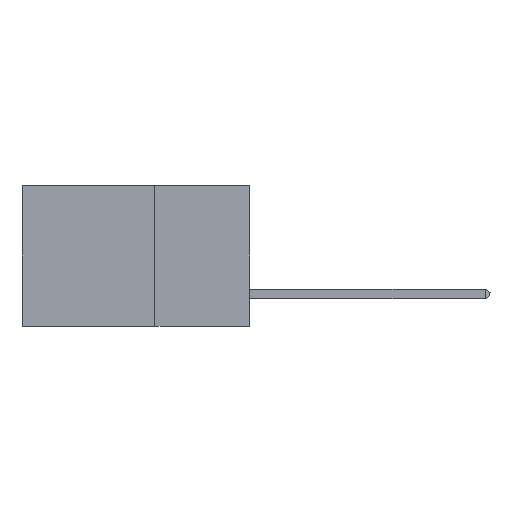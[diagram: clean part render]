
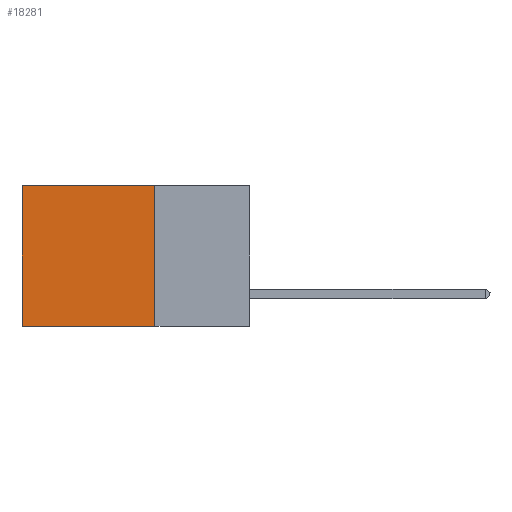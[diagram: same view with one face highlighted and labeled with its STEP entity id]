
A CAD part, left-side view. The second image highlights one B-rep face of the part: STEP entity #18281.
In plain terms, the highlighted planar face has unit normal (-1, 0, 0).
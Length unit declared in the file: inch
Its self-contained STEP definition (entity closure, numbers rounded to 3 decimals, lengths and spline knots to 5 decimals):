
#1124 = CARTESIAN_POINT ( 'NONE',  ( 0.2875, 0.6, 0. ) ) ;
#4220 = VERTEX_POINT ( 'NONE', #5582 ) ;
#4544 = VERTEX_POINT ( 'NONE', #17942 ) ;
#5419 = CARTESIAN_POINT ( 'NONE',  ( 0.2875, 0.25, 0. ) ) ;
#5428 = LINE ( 'NONE', #8437, #21747 ) ;
#5582 = CARTESIAN_POINT ( 'NONE',  ( 0.2875, 0.25, 0. ) ) ;
#7555 = VERTEX_POINT ( 'NONE', #14689 ) ;
#7795 = AXIS2_PLACEMENT_3D ( 'NONE', #24287, #32780, #15364 ) ;
#8168 = ORIENTED_EDGE ( 'NONE', *, *, #15503, .F. ) ;
#8437 = CARTESIAN_POINT ( 'NONE',  ( 0.2875, 0.25, 0. ) ) ;
#9145 = EDGE_LOOP ( 'NONE', ( #32439, #8168, #34085, #28938 ) ) ;
#14689 = CARTESIAN_POINT ( 'NONE',  ( 0.2875, 0.6, -0.37 ) ) ;
#14706 = FACE_OUTER_BOUND ( 'NONE', #9145, .T. ) ;
#14793 = EDGE_CURVE ( 'NONE', #4220, #32920, #35378, .T. ) ;
#15364 = DIRECTION ( 'NONE',  ( 0., 0., -1. ) ) ;
#15503 = EDGE_CURVE ( 'NONE', #32920, #7555, #32163, .T. ) ;
#17131 = CARTESIAN_POINT ( 'NONE',  ( 0.2875, 0.25, -0.37 ) ) ;
#17942 = CARTESIAN_POINT ( 'NONE',  ( 0.2875, 0.6, 0. ) ) ;
#18006 = VECTOR ( 'NONE', #20273, 39.37008 ) ;
#18010 = VECTOR ( 'NONE', #22036, 39.37008 ) ;
#18281 = ADVANCED_FACE ( 'NONE', ( #14706 ), #24543, .F. ) ;
#19982 = VECTOR ( 'NONE', #25679, 39.37008 ) ;
#20149 = DIRECTION ( 'NONE',  ( 0., 1., 0. ) ) ;
#20273 = DIRECTION ( 'NONE',  ( 0., 1., 0. ) ) ;
#21747 = VECTOR ( 'NONE', #20149, 39.37008 ) ;
#22036 = DIRECTION ( 'NONE',  ( 0., 0., -1. ) ) ;
#23110 = EDGE_CURVE ( 'NONE', #4220, #4544, #5428, .T. ) ;
#24287 = CARTESIAN_POINT ( 'NONE',  ( 0.2875, 0.25, 0. ) ) ;
#24543 = PLANE ( 'NONE',  #7795 ) ;
#25679 = DIRECTION ( 'NONE',  ( 0., 0., -1. ) ) ;
#28582 = LINE ( 'NONE', #1124, #18010 ) ;
#28938 = ORIENTED_EDGE ( 'NONE', *, *, #23110, .T. ) ;
#32163 = LINE ( 'NONE', #37586, #18006 ) ;
#32265 = EDGE_CURVE ( 'NONE', #4544, #7555, #28582, .T. ) ;
#32439 = ORIENTED_EDGE ( 'NONE', *, *, #32265, .T. ) ;
#32780 = DIRECTION ( 'NONE',  ( 1., 0., 0. ) ) ;
#32920 = VERTEX_POINT ( 'NONE', #17131 ) ;
#34085 = ORIENTED_EDGE ( 'NONE', *, *, #14793, .F. ) ;
#35378 = LINE ( 'NONE', #5419, #19982 ) ;
#37586 = CARTESIAN_POINT ( 'NONE',  ( 0.2875, 0.25, -0.37 ) ) ;
